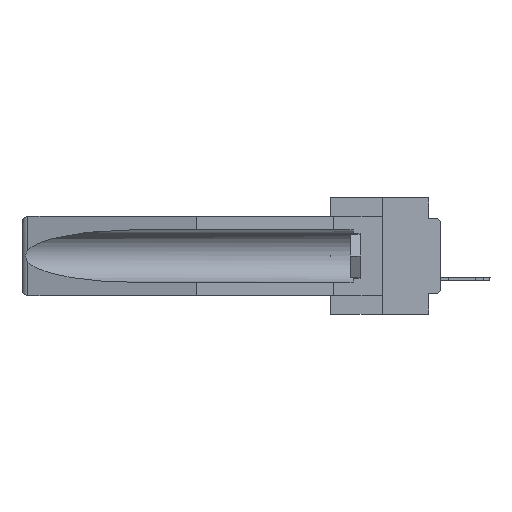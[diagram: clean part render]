
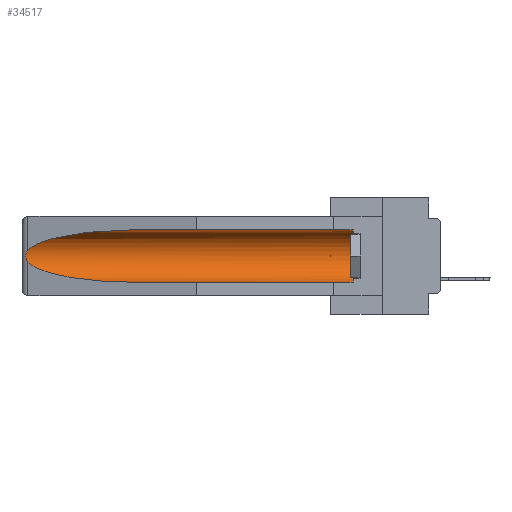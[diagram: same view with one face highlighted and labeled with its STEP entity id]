
A CAD part, left-side view. The second image highlights one B-rep face of the part: STEP entity #34517.
In plain terms, the highlighted cylindrical face has radius 2.857 mm (diameter 5.715 mm), a partial arc.
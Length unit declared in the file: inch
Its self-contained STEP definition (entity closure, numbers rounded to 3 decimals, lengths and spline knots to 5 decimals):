
#42 = ORIENTED_EDGE ( 'NONE', *, *, #39085, .T. ) ;
#1010 = CARTESIAN_POINT ( 'NONE',  ( 0.155, -0.30754, -0.1715 ) ) ;
#1947 = CARTESIAN_POINT ( 'NONE',  ( 0.26597, 1.52961, -0.15275 ) ) ;
#2071 = EDGE_LOOP ( 'NONE', ( #18405, #42, #36212, #12190, #8017, #25082 ) ) ;
#2082 = CARTESIAN_POINT ( 'NONE',  ( 0.26654, 1.53092, -0.15636 ) ) ;
#2132 = AXIS2_PLACEMENT_3D ( 'NONE', #37648, #10862, #37932 ) ;
#2221 = CARTESIAN_POINT ( 'NONE',  ( 0.155, 0.126, -0.059 ) ) ;
#3071 = VECTOR ( 'NONE', #37477, 39.37008 ) ;
#3296 = B_SPLINE_CURVE_WITH_KNOTS ( 'NONE', 3,
 ( #38228, #1947, #2082, #38367, #20150, #23333, #5052, #23601, #17632, #26303 ),
 .UNSPECIFIED., .F., .F.,
 ( 4, 2, 2, 2, 4 ),
 ( 0., 0.00029, 0.00058, 0.00087, 0.00117 ),
 .UNSPECIFIED. ) ;
#4490 = CARTESIAN_POINT ( 'NONE',  ( 0.26537, 1.52718, -0.19328 ) ) ;
#5052 = CARTESIAN_POINT ( 'NONE',  ( 0.2673, 1.53269, -0.17917 ) ) ;
#6575 = CARTESIAN_POINT ( 'NONE',  ( 0.26537, 1.52718, -0.14972 ) ) ;
#8017 = ORIENTED_EDGE ( 'NONE', *, *, #25950, .T. ) ;
#9024 = VERTEX_POINT ( 'NONE', #2221 ) ;
#10384 = CARTESIAN_POINT ( 'NONE',  ( 0.26537, 1.52718, -0.19328 ) ) ;
#10862 = DIRECTION ( 'NONE',  ( 0., -1., 0. ) ) ;
#10970 = VERTEX_POINT ( 'NONE', #11368 ) ;
#11368 = CARTESIAN_POINT ( 'NONE',  ( 0.155, 1.07973, -0.284 ) ) ;
#11990 = VERTEX_POINT ( 'NONE', #32469 ) ;
#12190 = ORIENTED_EDGE ( 'NONE', *, *, #23018, .F. ) ;
#12732 =( BOUNDED_CURVE ( )  B_SPLINE_CURVE ( 3, ( #10384, #16203, #25304, #19244 ),
 .UNSPECIFIED., .F., .F. ) 
 B_SPLINE_CURVE_WITH_KNOTS ( ( 4, 4 ),
 ( 0.1948, 1.5708 ),
 .UNSPECIFIED. ) 
 CURVE ( )  GEOMETRIC_REPRESENTATION_ITEM ( )  RATIONAL_B_SPLINE_CURVE ( ( 1., 0.848, 0.848, 1. ) ) 
 REPRESENTATION_ITEM ( '' )  );
#13108 = DIRECTION ( 'NONE',  ( 0., 0., 1. ) ) ;
#13303 = CARTESIAN_POINT ( 'NONE',  ( 0.155, -0.30754, -0.059 ) ) ;
#16203 = CARTESIAN_POINT ( 'NONE',  ( 0.25451, 1.48313, -0.24835 ) ) ;
#16902 =( BOUNDED_CURVE ( )  B_SPLINE_CURVE ( 3, ( #33496, #18368, #24337, #6575 ),
 .UNSPECIFIED., .F., .F. ) 
 B_SPLINE_CURVE_WITH_KNOTS ( ( 4, 4 ),
 ( 4.71239, 6.08839 ),
 .UNSPECIFIED. ) 
 CURVE ( )  GEOMETRIC_REPRESENTATION_ITEM ( )  RATIONAL_B_SPLINE_CURVE ( ( 1., 0.848, 0.848, 1. ) ) 
 REPRESENTATION_ITEM ( '' )  );
#17632 = CARTESIAN_POINT ( 'NONE',  ( 0.26597, 1.5296, -0.19026 ) ) ;
#18368 = CARTESIAN_POINT ( 'NONE',  ( 0.21114, 1.30732, -0.059 ) ) ;
#18405 = ORIENTED_EDGE ( 'NONE', *, *, #31720, .T. ) ;
#19244 = CARTESIAN_POINT ( 'NONE',  ( 0.155, 1.07973, -0.284 ) ) ;
#20150 = CARTESIAN_POINT ( 'NONE',  ( 0.2675, 1.53308, -0.16763 ) ) ;
#21501 = FACE_OUTER_BOUND ( 'NONE', #2071, .T. ) ;
#21915 = CYLINDRICAL_SURFACE ( 'NONE', #31475, 0.1125 ) ;
#23018 = EDGE_CURVE ( 'NONE', #35357, #10970, #26758, .T. ) ;
#23303 = CIRCLE ( 'NONE', #2132, 0.1125 ) ;
#23333 = CARTESIAN_POINT ( 'NONE',  ( 0.2675, 1.53308, -0.17534 ) ) ;
#23601 = CARTESIAN_POINT ( 'NONE',  ( 0.26655, 1.53094, -0.18657 ) ) ;
#23612 = EDGE_CURVE ( 'NONE', #9024, #11990, #30043, .T. ) ;
#24337 = CARTESIAN_POINT ( 'NONE',  ( 0.25451, 1.48313, -0.09465 ) ) ;
#25082 = ORIENTED_EDGE ( 'NONE', *, *, #23612, .T. ) ;
#25304 = CARTESIAN_POINT ( 'NONE',  ( 0.21114, 1.30732, -0.284 ) ) ;
#25950 = EDGE_CURVE ( 'NONE', #35357, #9024, #23303, .T. ) ;
#26303 = CARTESIAN_POINT ( 'NONE',  ( 0.26537, 1.52718, -0.19328 ) ) ;
#26758 = LINE ( 'NONE', #31776, #35729 ) ;
#27575 = VERTEX_POINT ( 'NONE', #4490 ) ;
#28572 = CARTESIAN_POINT ( 'NONE',  ( 0.26537, 1.52718, -0.14972 ) ) ;
#28667 = VERTEX_POINT ( 'NONE', #28572 ) ;
#30043 = LINE ( 'NONE', #13303, #3071 ) ;
#30215 = EDGE_CURVE ( 'NONE', #27575, #10970, #12732, .T. ) ;
#31475 = AXIS2_PLACEMENT_3D ( 'NONE', #1010, #37416, #13108 ) ;
#31720 = EDGE_CURVE ( 'NONE', #11990, #28667, #16902, .T. ) ;
#31776 = CARTESIAN_POINT ( 'NONE',  ( 0.155, -0.30754, -0.284 ) ) ;
#32469 = CARTESIAN_POINT ( 'NONE',  ( 0.155, 1.07973, -0.059 ) ) ;
#33496 = CARTESIAN_POINT ( 'NONE',  ( 0.155, 1.07973, -0.059 ) ) ;
#34517 = ADVANCED_FACE ( 'NONE', ( #21501 ), #21915, .F. ) ;
#35079 = DIRECTION ( 'NONE',  ( 0., 1., 0. ) ) ;
#35357 = VERTEX_POINT ( 'NONE', #38643 ) ;
#35729 = VECTOR ( 'NONE', #35079, 39.37008 ) ;
#36212 = ORIENTED_EDGE ( 'NONE', *, *, #30215, .T. ) ;
#37416 = DIRECTION ( 'NONE',  ( 0., 1., 0. ) ) ;
#37477 = DIRECTION ( 'NONE',  ( 0., 1., 0. ) ) ;
#37648 = CARTESIAN_POINT ( 'NONE',  ( 0.155, 0.126, -0.1715 ) ) ;
#37932 = DIRECTION ( 'NONE',  ( 0., 0., 1. ) ) ;
#38228 = CARTESIAN_POINT ( 'NONE',  ( 0.26537, 1.52718, -0.14972 ) ) ;
#38367 = CARTESIAN_POINT ( 'NONE',  ( 0.2673, 1.5327, -0.16383 ) ) ;
#38643 = CARTESIAN_POINT ( 'NONE',  ( 0.155, 0.126, -0.284 ) ) ;
#39085 = EDGE_CURVE ( 'NONE', #28667, #27575, #3296, .T. ) ;
